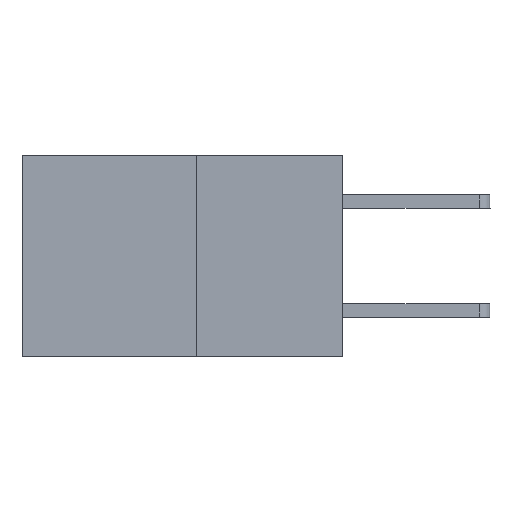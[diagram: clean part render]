
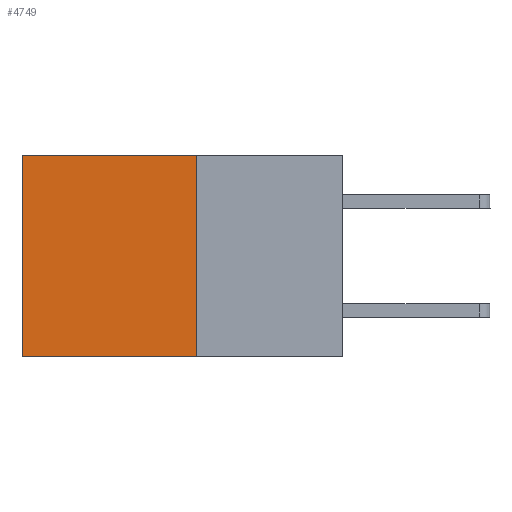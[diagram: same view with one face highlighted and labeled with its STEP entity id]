
A CAD part, left-side view. The second image highlights one B-rep face of the part: STEP entity #4749.
In plain terms, the highlighted planar face has unit normal (-1, 0, 0).
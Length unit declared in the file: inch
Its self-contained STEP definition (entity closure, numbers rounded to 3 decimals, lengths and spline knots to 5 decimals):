
#8 = VECTOR ( 'NONE', #1368, 39.37008 ) ;
#457 = LINE ( 'NONE', #2403, #8 ) ;
#662 = LINE ( 'NONE', #2483, #6965 ) ;
#742 = VECTOR ( 'NONE', #3431, 39.37008 ) ;
#1003 = DIRECTION ( 'NONE',  ( 0., 0., -1. ) ) ;
#1164 = EDGE_CURVE ( 'NONE', #6518, #5272, #662, .T. ) ;
#1206 = EDGE_CURVE ( 'NONE', #4937, #5272, #457, .T. ) ;
#1368 = DIRECTION ( 'NONE',  ( 0., 0., -1. ) ) ;
#1705 = ORIENTED_EDGE ( 'NONE', *, *, #1164, .F. ) ;
#1883 = VERTEX_POINT ( 'NONE', #5179 ) ;
#2397 = AXIS2_PLACEMENT_3D ( 'NONE', #4767, #4298, #4240 ) ;
#2403 = CARTESIAN_POINT ( 'NONE',  ( 0.277, 0.59, -0.37 ) ) ;
#2483 = CARTESIAN_POINT ( 'NONE',  ( 0.277, 0.27, -0.37 ) ) ;
#2853 = CARTESIAN_POINT ( 'NONE',  ( 0.277, 0.27, -0.37 ) ) ;
#3247 = FACE_OUTER_BOUND ( 'NONE', #6845, .T. ) ;
#3284 = ORIENTED_EDGE ( 'NONE', *, *, #1206, .T. ) ;
#3431 = DIRECTION ( 'NONE',  ( 0., 1., 0. ) ) ;
#3466 = CARTESIAN_POINT ( 'NONE',  ( 0.277, 0.27, 0. ) ) ;
#3667 = LINE ( 'NONE', #2853, #5236 ) ;
#4179 = PLANE ( 'NONE',  #2397 ) ;
#4240 = DIRECTION ( 'NONE',  ( 0., 0., -1. ) ) ;
#4298 = DIRECTION ( 'NONE',  ( 1., 0., 0. ) ) ;
#4326 = CARTESIAN_POINT ( 'NONE',  ( 0.277, 0.59, 0. ) ) ;
#4458 = DIRECTION ( 'NONE',  ( 0., 1., 0. ) ) ;
#4749 = ADVANCED_FACE ( 'NONE', ( #3247 ), #4179, .F. ) ;
#4767 = CARTESIAN_POINT ( 'NONE',  ( 0.277, 0.27, -0.37 ) ) ;
#4937 = VERTEX_POINT ( 'NONE', #4326 ) ;
#5064 = ORIENTED_EDGE ( 'NONE', *, *, #5793, .F. ) ;
#5179 = CARTESIAN_POINT ( 'NONE',  ( 0.277, 0.27, 0. ) ) ;
#5236 = VECTOR ( 'NONE', #1003, 39.37008 ) ;
#5270 = ORIENTED_EDGE ( 'NONE', *, *, #7245, .T. ) ;
#5272 = VERTEX_POINT ( 'NONE', #7065 ) ;
#5793 = EDGE_CURVE ( 'NONE', #1883, #6518, #3667, .T. ) ;
#6518 = VERTEX_POINT ( 'NONE', #8025 ) ;
#6845 = EDGE_LOOP ( 'NONE', ( #3284, #1705, #5064, #5270 ) ) ;
#6965 = VECTOR ( 'NONE', #4458, 39.37008 ) ;
#7065 = CARTESIAN_POINT ( 'NONE',  ( 0.277, 0.59, -0.37 ) ) ;
#7245 = EDGE_CURVE ( 'NONE', #1883, #4937, #7626, .T. ) ;
#7626 = LINE ( 'NONE', #3466, #742 ) ;
#8025 = CARTESIAN_POINT ( 'NONE',  ( 0.277, 0.27, -0.37 ) ) ;
